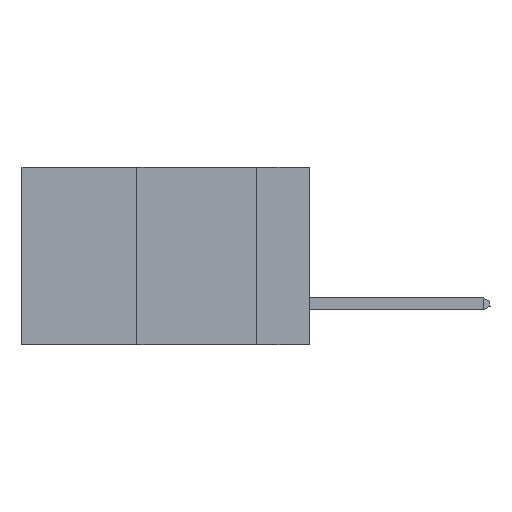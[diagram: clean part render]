
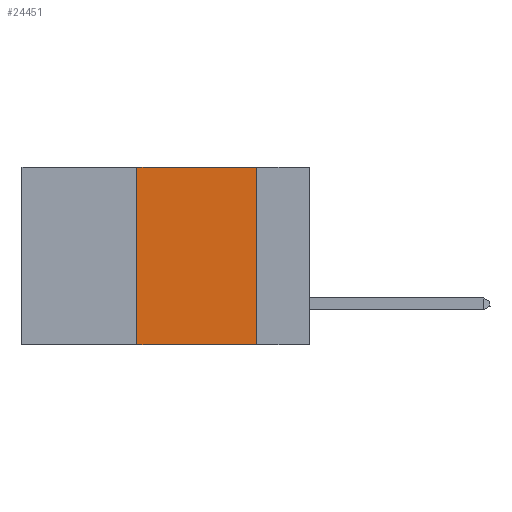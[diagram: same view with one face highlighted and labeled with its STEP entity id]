
A CAD part, left-side view. The second image highlights one B-rep face of the part: STEP entity #24451.
In plain terms, the highlighted planar face has unit normal (-1, 0, 0).
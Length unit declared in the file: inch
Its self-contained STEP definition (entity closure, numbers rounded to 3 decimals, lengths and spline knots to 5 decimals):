
#472 = EDGE_CURVE ( 'NONE', #26986, #13165, #5427, .T. ) ;
#713 = VECTOR ( 'NONE', #27649, 39.37008 ) ;
#1237 = EDGE_CURVE ( 'NONE', #13165, #6983, #28909, .T. ) ;
#1865 = CARTESIAN_POINT ( 'NONE',  ( 0., 0.6, -0.37 ) ) ;
#3039 = LINE ( 'NONE', #1865, #22412 ) ;
#3635 = DIRECTION ( 'NONE',  ( 0., -1., 0. ) ) ;
#3752 = CARTESIAN_POINT ( 'NONE',  ( 0., 0.36, 0. ) ) ;
#4441 = EDGE_LOOP ( 'NONE', ( #31374, #24970, #8350, #25690 ) ) ;
#5427 = LINE ( 'NONE', #24886, #18520 ) ;
#6983 = VERTEX_POINT ( 'NONE', #28859 ) ;
#8249 = CARTESIAN_POINT ( 'NONE',  ( 0., 0.6, 0. ) ) ;
#8350 = ORIENTED_EDGE ( 'NONE', *, *, #11545, .F. ) ;
#10404 = VERTEX_POINT ( 'NONE', #24855 ) ;
#11545 = EDGE_CURVE ( 'NONE', #10404, #26986, #26165, .T. ) ;
#13165 = VERTEX_POINT ( 'NONE', #23796 ) ;
#14152 = EDGE_CURVE ( 'NONE', #10404, #6983, #3039, .T. ) ;
#15325 = AXIS2_PLACEMENT_3D ( 'NONE', #8249, #23648, #16496 ) ;
#16496 = DIRECTION ( 'NONE',  ( 0., 0., -1. ) ) ;
#18009 = DIRECTION ( 'NONE',  ( 0., -1., 0. ) ) ;
#18520 = VECTOR ( 'NONE', #3635, 39.37008 ) ;
#18991 = VECTOR ( 'NONE', #24079, 39.37008 ) ;
#19881 = CARTESIAN_POINT ( 'NONE',  ( 0., 0.36, 0. ) ) ;
#22412 = VECTOR ( 'NONE', #18009, 39.37008 ) ;
#23648 = DIRECTION ( 'NONE',  ( 1., 0., 0. ) ) ;
#23796 = CARTESIAN_POINT ( 'NONE',  ( 0., 0.11, 0. ) ) ;
#24079 = DIRECTION ( 'NONE',  ( 0., 0., 1. ) ) ;
#24342 = PLANE ( 'NONE',  #15325 ) ;
#24451 = ADVANCED_FACE ( 'NONE', ( #31310 ), #24342, .F. ) ;
#24855 = CARTESIAN_POINT ( 'NONE',  ( 0., 0.36, -0.37 ) ) ;
#24886 = CARTESIAN_POINT ( 'NONE',  ( 0., 0.6, 0. ) ) ;
#24970 = ORIENTED_EDGE ( 'NONE', *, *, #472, .F. ) ;
#25690 = ORIENTED_EDGE ( 'NONE', *, *, #14152, .T. ) ;
#26165 = LINE ( 'NONE', #19881, #18991 ) ;
#26986 = VERTEX_POINT ( 'NONE', #3752 ) ;
#27649 = DIRECTION ( 'NONE',  ( 0., 0., -1. ) ) ;
#28859 = CARTESIAN_POINT ( 'NONE',  ( 0., 0.11, -0.37 ) ) ;
#28909 = LINE ( 'NONE', #31975, #713 ) ;
#31310 = FACE_OUTER_BOUND ( 'NONE', #4441, .T. ) ;
#31374 = ORIENTED_EDGE ( 'NONE', *, *, #1237, .F. ) ;
#31975 = CARTESIAN_POINT ( 'NONE',  ( 0., 0.11, 0. ) ) ;
